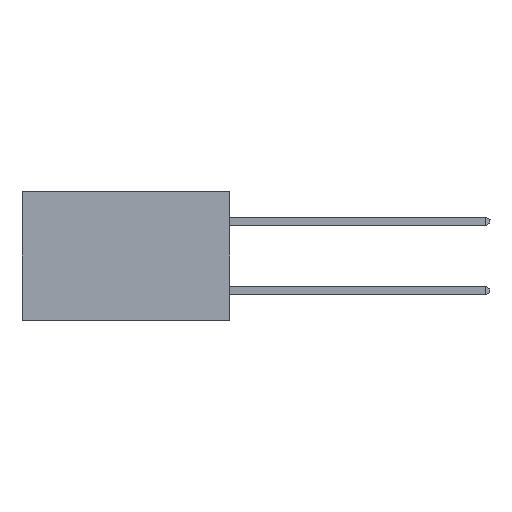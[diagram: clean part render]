
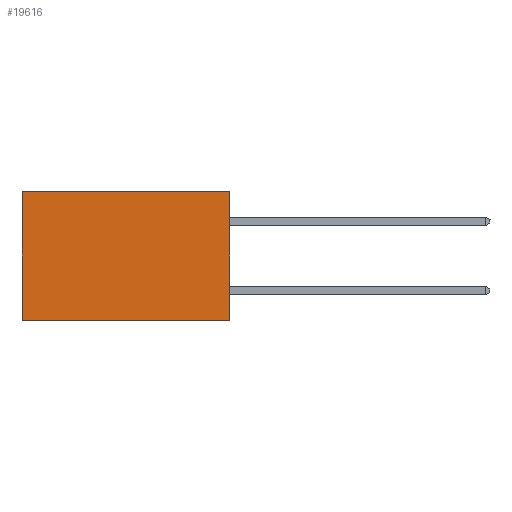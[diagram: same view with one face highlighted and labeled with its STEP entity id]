
A CAD part, left-side view. The second image highlights one B-rep face of the part: STEP entity #19616.
In plain terms, the highlighted planar face has unit normal (-1, 0, 0).
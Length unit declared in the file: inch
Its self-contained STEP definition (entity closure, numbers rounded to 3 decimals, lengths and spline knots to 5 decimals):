
#2921 = CARTESIAN_POINT ( 'NONE',  ( 0.298, 0., 0. ) ) ;
#2973 = EDGE_CURVE ( 'NONE', #22605, #19297, #21200, .T. ) ;
#3638 = DIRECTION ( 'NONE',  ( 0., 0., -1. ) ) ;
#4072 = DIRECTION ( 'NONE',  ( 0., 1., 0. ) ) ;
#4530 = CARTESIAN_POINT ( 'NONE',  ( 0.298, 0.6, 0. ) ) ;
#5482 = CARTESIAN_POINT ( 'NONE',  ( 0.298, 0., -0.37 ) ) ;
#5515 = CARTESIAN_POINT ( 'NONE',  ( 0.298, 0.6, -0.37 ) ) ;
#7245 = DIRECTION ( 'NONE',  ( 0., 1., 0. ) ) ;
#7878 = EDGE_LOOP ( 'NONE', ( #13525, #21129, #10402, #19939 ) ) ;
#8035 = EDGE_CURVE ( 'NONE', #18009, #9958, #16133, .T. ) ;
#9958 = VERTEX_POINT ( 'NONE', #17505 ) ;
#10402 = ORIENTED_EDGE ( 'NONE', *, *, #12912, .F. ) ;
#11607 = LINE ( 'NONE', #14704, #13882 ) ;
#12912 = EDGE_CURVE ( 'NONE', #18009, #22605, #11607, .T. ) ;
#13525 = ORIENTED_EDGE ( 'NONE', *, *, #14185, .T. ) ;
#13882 = VECTOR ( 'NONE', #3638, 39.37008 ) ;
#14185 = EDGE_CURVE ( 'NONE', #9958, #19297, #15929, .T. ) ;
#14478 = CARTESIAN_POINT ( 'NONE',  ( 0.298, 0., 0. ) ) ;
#14567 = DIRECTION ( 'NONE',  ( 1., 0., 0. ) ) ;
#14704 = CARTESIAN_POINT ( 'NONE',  ( 0.298, 0., 0. ) ) ;
#15929 = LINE ( 'NONE', #4530, #17361 ) ;
#16133 = LINE ( 'NONE', #20076, #23666 ) ;
#16350 = DIRECTION ( 'NONE',  ( 0., 0., -1. ) ) ;
#16984 = CARTESIAN_POINT ( 'NONE',  ( 0.298, 0., -0.37 ) ) ;
#17236 = AXIS2_PLACEMENT_3D ( 'NONE', #14478, #14567, #16350 ) ;
#17361 = VECTOR ( 'NONE', #21332, 39.37008 ) ;
#17505 = CARTESIAN_POINT ( 'NONE',  ( 0.298, 0.6, 0. ) ) ;
#17717 = FACE_OUTER_BOUND ( 'NONE', #7878, .T. ) ;
#18009 = VERTEX_POINT ( 'NONE', #2921 ) ;
#19297 = VERTEX_POINT ( 'NONE', #5515 ) ;
#19616 = ADVANCED_FACE ( 'NONE', ( #17717 ), #23723, .F. ) ;
#19939 = ORIENTED_EDGE ( 'NONE', *, *, #8035, .T. ) ;
#20076 = CARTESIAN_POINT ( 'NONE',  ( 0.298, 0., 0. ) ) ;
#20914 = VECTOR ( 'NONE', #4072, 39.37008 ) ;
#21129 = ORIENTED_EDGE ( 'NONE', *, *, #2973, .F. ) ;
#21200 = LINE ( 'NONE', #16984, #20914 ) ;
#21332 = DIRECTION ( 'NONE',  ( 0., 0., -1. ) ) ;
#22605 = VERTEX_POINT ( 'NONE', #5482 ) ;
#23666 = VECTOR ( 'NONE', #7245, 39.37008 ) ;
#23723 = PLANE ( 'NONE',  #17236 ) ;
